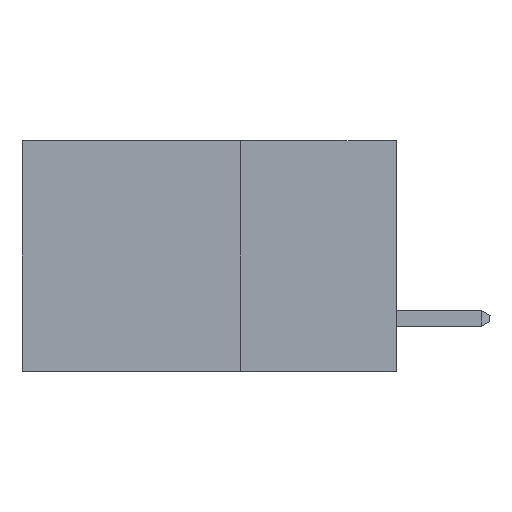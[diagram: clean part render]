
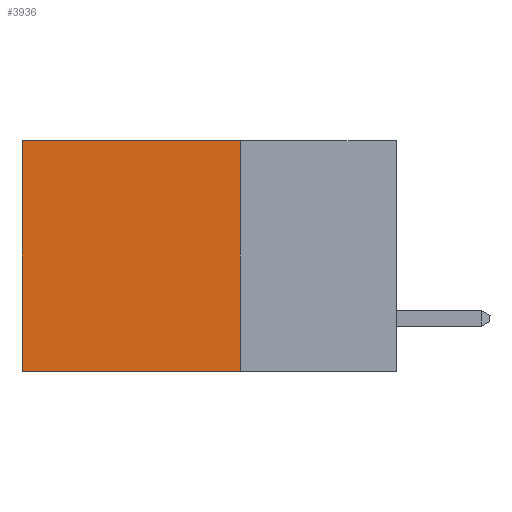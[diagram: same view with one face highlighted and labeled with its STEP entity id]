
A CAD part, left-side view. The second image highlights one B-rep face of the part: STEP entity #3936.
In plain terms, the highlighted planar face has unit normal (-1, 0, 0).
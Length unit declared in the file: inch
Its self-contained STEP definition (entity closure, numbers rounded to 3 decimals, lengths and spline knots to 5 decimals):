
#558 = EDGE_LOOP ( 'NONE', ( #2941, #13678, #13897, #16236 ) ) ;
#1784 = AXIS2_PLACEMENT_3D ( 'NONE', #12900, #14289, #13006 ) ;
#2574 = CARTESIAN_POINT ( 'NONE',  ( 0.298, 0.25, 0. ) ) ;
#2941 = ORIENTED_EDGE ( 'NONE', *, *, #7472, .T. ) ;
#3113 = VERTEX_POINT ( 'NONE', #2574 ) ;
#3747 = DIRECTION ( 'NONE',  ( 0., 1., 0. ) ) ;
#3850 = EDGE_CURVE ( 'NONE', #3113, #15104, #11800, .T. ) ;
#3936 = ADVANCED_FACE ( 'NONE', ( #10143 ), #12628, .F. ) ;
#4507 = EDGE_CURVE ( 'NONE', #3113, #16617, #11387, .T. ) ;
#5182 = CARTESIAN_POINT ( 'NONE',  ( 0.298, 0.25, 0. ) ) ;
#6299 = CARTESIAN_POINT ( 'NONE',  ( 0.298, 0.6, -0.37 ) ) ;
#6524 = VECTOR ( 'NONE', #12057, 39.37008 ) ;
#6591 = CARTESIAN_POINT ( 'NONE',  ( 0.298, 0.6, 0. ) ) ;
#7472 = EDGE_CURVE ( 'NONE', #16617, #11052, #11280, .T. ) ;
#7827 = VECTOR ( 'NONE', #3747, 39.37008 ) ;
#8265 = VECTOR ( 'NONE', #14008, 39.37008 ) ;
#8787 = LINE ( 'NONE', #10249, #6524 ) ;
#9317 = DIRECTION ( 'NONE',  ( 0., 0., -1. ) ) ;
#9394 = VECTOR ( 'NONE', #9317, 39.37008 ) ;
#10143 = FACE_OUTER_BOUND ( 'NONE', #558, .T. ) ;
#10249 = CARTESIAN_POINT ( 'NONE',  ( 0.298, 0.25, -0.37 ) ) ;
#10760 = EDGE_CURVE ( 'NONE', #15104, #11052, #8787, .T. ) ;
#11052 = VERTEX_POINT ( 'NONE', #6299 ) ;
#11280 = LINE ( 'NONE', #11930, #9394 ) ;
#11387 = LINE ( 'NONE', #5182, #7827 ) ;
#11800 = LINE ( 'NONE', #15425, #8265 ) ;
#11930 = CARTESIAN_POINT ( 'NONE',  ( 0.298, 0.6, 0. ) ) ;
#12057 = DIRECTION ( 'NONE',  ( 0., 1., 0. ) ) ;
#12058 = CARTESIAN_POINT ( 'NONE',  ( 0.298, 0.25, -0.37 ) ) ;
#12628 = PLANE ( 'NONE',  #1784 ) ;
#12900 = CARTESIAN_POINT ( 'NONE',  ( 0.298, 0.25, 0. ) ) ;
#13006 = DIRECTION ( 'NONE',  ( 0., 0., -1. ) ) ;
#13678 = ORIENTED_EDGE ( 'NONE', *, *, #10760, .F. ) ;
#13897 = ORIENTED_EDGE ( 'NONE', *, *, #3850, .F. ) ;
#14008 = DIRECTION ( 'NONE',  ( 0., 0., -1. ) ) ;
#14289 = DIRECTION ( 'NONE',  ( 1., 0., 0. ) ) ;
#15104 = VERTEX_POINT ( 'NONE', #12058 ) ;
#15425 = CARTESIAN_POINT ( 'NONE',  ( 0.298, 0.25, 0. ) ) ;
#16236 = ORIENTED_EDGE ( 'NONE', *, *, #4507, .T. ) ;
#16617 = VERTEX_POINT ( 'NONE', #6591 ) ;
